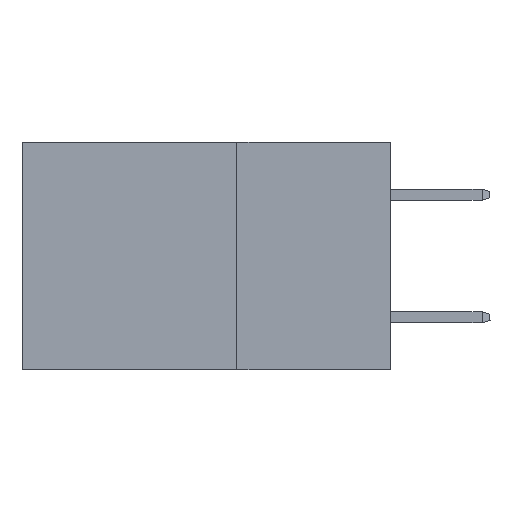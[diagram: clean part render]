
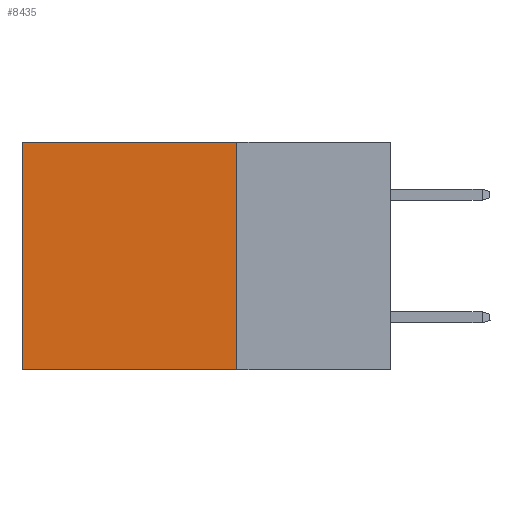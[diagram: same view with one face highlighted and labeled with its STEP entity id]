
A CAD part, left-side view. The second image highlights one B-rep face of the part: STEP entity #8435.
In plain terms, the highlighted planar face has unit normal (-1, 0, 0).
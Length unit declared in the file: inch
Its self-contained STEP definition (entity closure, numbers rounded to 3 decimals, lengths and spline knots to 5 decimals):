
#15 = VERTEX_POINT ( 'NONE', #13219 ) ;
#747 = CARTESIAN_POINT ( 'NONE',  ( 0.2875, 0.25, 0. ) ) ;
#1016 = DIRECTION ( 'NONE',  ( 0., 1., 0. ) ) ;
#1526 = VECTOR ( 'NONE', #1016, 39.37008 ) ;
#1945 = CARTESIAN_POINT ( 'NONE',  ( 0.2875, 0.6, 0. ) ) ;
#2219 = DIRECTION ( 'NONE',  ( 0., 0., -1. ) ) ;
#3102 = EDGE_LOOP ( 'NONE', ( #11481, #16601, #11998, #17484 ) ) ;
#3222 = CARTESIAN_POINT ( 'NONE',  ( 0.2875, 0.25, 0. ) ) ;
#3520 = EDGE_CURVE ( 'NONE', #16071, #15969, #6983, .T. ) ;
#6907 = EDGE_CURVE ( 'NONE', #15969, #7081, #23045, .T. ) ;
#6983 = LINE ( 'NONE', #747, #1526 ) ;
#7081 = VERTEX_POINT ( 'NONE', #14249 ) ;
#7815 = VECTOR ( 'NONE', #2219, 39.37008 ) ;
#8435 = ADVANCED_FACE ( 'NONE', ( #9623 ), #16530, .F. ) ;
#9623 = FACE_OUTER_BOUND ( 'NONE', #3102, .T. ) ;
#9872 = CARTESIAN_POINT ( 'NONE',  ( 0.2875, 0.25, 0. ) ) ;
#10508 = VECTOR ( 'NONE', #18378, 39.37008 ) ;
#11481 = ORIENTED_EDGE ( 'NONE', *, *, #6907, .T. ) ;
#11998 = ORIENTED_EDGE ( 'NONE', *, *, #15373, .F. ) ;
#12362 = LINE ( 'NONE', #21985, #10508 ) ;
#13219 = CARTESIAN_POINT ( 'NONE',  ( 0.2875, 0.25, -0.37 ) ) ;
#14249 = CARTESIAN_POINT ( 'NONE',  ( 0.2875, 0.6, -0.37 ) ) ;
#14935 = DIRECTION ( 'NONE',  ( 1., 0., 0. ) ) ;
#15201 = VECTOR ( 'NONE', #20981, 39.37008 ) ;
#15373 = EDGE_CURVE ( 'NONE', #16071, #15, #25123, .T. ) ;
#15969 = VERTEX_POINT ( 'NONE', #1945 ) ;
#16071 = VERTEX_POINT ( 'NONE', #9872 ) ;
#16530 = PLANE ( 'NONE',  #18056 ) ;
#16601 = ORIENTED_EDGE ( 'NONE', *, *, #20188, .F. ) ;
#17484 = ORIENTED_EDGE ( 'NONE', *, *, #3520, .T. ) ;
#18056 = AXIS2_PLACEMENT_3D ( 'NONE', #3222, #14935, #20405 ) ;
#18378 = DIRECTION ( 'NONE',  ( 0., 1., 0. ) ) ;
#19635 = CARTESIAN_POINT ( 'NONE',  ( 0.2875, 0.6, 0. ) ) ;
#20188 = EDGE_CURVE ( 'NONE', #15, #7081, #12362, .T. ) ;
#20405 = DIRECTION ( 'NONE',  ( 0., 0., -1. ) ) ;
#20981 = DIRECTION ( 'NONE',  ( 0., 0., -1. ) ) ;
#21985 = CARTESIAN_POINT ( 'NONE',  ( 0.2875, 0.25, -0.37 ) ) ;
#23045 = LINE ( 'NONE', #19635, #15201 ) ;
#23439 = CARTESIAN_POINT ( 'NONE',  ( 0.2875, 0.25, 0. ) ) ;
#25123 = LINE ( 'NONE', #23439, #7815 ) ;
